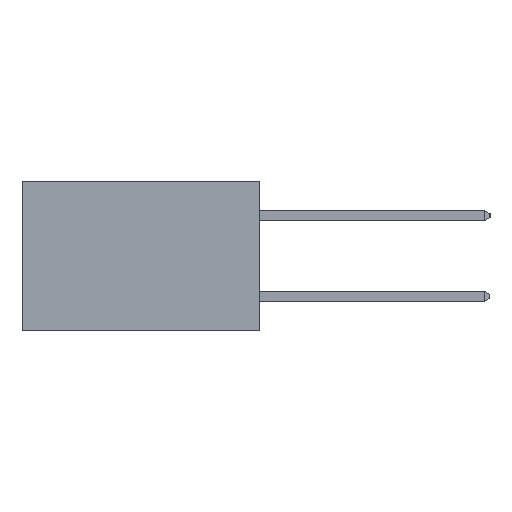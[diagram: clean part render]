
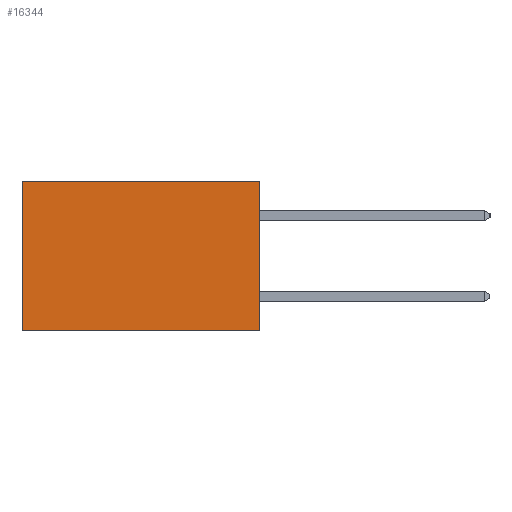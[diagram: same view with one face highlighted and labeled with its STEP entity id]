
A CAD part, left-side view. The second image highlights one B-rep face of the part: STEP entity #16344.
In plain terms, the highlighted planar face has unit normal (-1, 0, 0).
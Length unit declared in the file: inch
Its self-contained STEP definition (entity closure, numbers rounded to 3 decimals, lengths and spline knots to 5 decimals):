
#180 = VECTOR ( 'NONE', #19115, 39.37008 ) ;
#1066 = CARTESIAN_POINT ( 'NONE',  ( 0.277, 0.59, -0.37 ) ) ;
#2022 = VERTEX_POINT ( 'NONE', #5059 ) ;
#2050 = ORIENTED_EDGE ( 'NONE', *, *, #21146, .T. ) ;
#2096 = CARTESIAN_POINT ( 'NONE',  ( 0.277, 0., -0.37 ) ) ;
#2317 = DIRECTION ( 'NONE',  ( 1., 0., 0. ) ) ;
#2644 = ORIENTED_EDGE ( 'NONE', *, *, #7442, .F. ) ;
#2750 = ORIENTED_EDGE ( 'NONE', *, *, #17322, .F. ) ;
#3380 = LINE ( 'NONE', #2096, #12938 ) ;
#3506 = DIRECTION ( 'NONE',  ( 0., 1., 0. ) ) ;
#4027 = ORIENTED_EDGE ( 'NONE', *, *, #23613, .T. ) ;
#5059 = CARTESIAN_POINT ( 'NONE',  ( 0.277, 0.59, 0. ) ) ;
#5318 = LINE ( 'NONE', #1066, #19047 ) ;
#7302 = CARTESIAN_POINT ( 'NONE',  ( 0.277, 0., 0. ) ) ;
#7442 = EDGE_CURVE ( 'NONE', #10250, #15735, #20271, .T. ) ;
#9732 = DIRECTION ( 'NONE',  ( 0., 0., -1. ) ) ;
#9875 = CARTESIAN_POINT ( 'NONE',  ( 0.277, 0., -0.37 ) ) ;
#10025 = VECTOR ( 'NONE', #3506, 39.37008 ) ;
#10250 = VERTEX_POINT ( 'NONE', #10329 ) ;
#10329 = CARTESIAN_POINT ( 'NONE',  ( 0.277, 0., -0.37 ) ) ;
#11353 = AXIS2_PLACEMENT_3D ( 'NONE', #13780, #2317, #15671 ) ;
#12938 = VECTOR ( 'NONE', #9732, 39.37008 ) ;
#13780 = CARTESIAN_POINT ( 'NONE',  ( 0.277, 0., -0.37 ) ) ;
#15092 = LINE ( 'NONE', #7302, #10025 ) ;
#15671 = DIRECTION ( 'NONE',  ( 0., 0., -1. ) ) ;
#15735 = VERTEX_POINT ( 'NONE', #22852 ) ;
#15897 = FACE_OUTER_BOUND ( 'NONE', #21923, .T. ) ;
#16344 = ADVANCED_FACE ( 'NONE', ( #15897 ), #22672, .F. ) ;
#16365 = DIRECTION ( 'NONE',  ( 0., 0., -1. ) ) ;
#17322 = EDGE_CURVE ( 'NONE', #20173, #10250, #3380, .T. ) ;
#17335 = CARTESIAN_POINT ( 'NONE',  ( 0.277, 0., 0. ) ) ;
#19047 = VECTOR ( 'NONE', #16365, 39.37008 ) ;
#19115 = DIRECTION ( 'NONE',  ( 0., 1., 0. ) ) ;
#20173 = VERTEX_POINT ( 'NONE', #17335 ) ;
#20271 = LINE ( 'NONE', #9875, #180 ) ;
#21146 = EDGE_CURVE ( 'NONE', #2022, #15735, #5318, .T. ) ;
#21923 = EDGE_LOOP ( 'NONE', ( #2050, #2644, #2750, #4027 ) ) ;
#22672 = PLANE ( 'NONE',  #11353 ) ;
#22852 = CARTESIAN_POINT ( 'NONE',  ( 0.277, 0.59, -0.37 ) ) ;
#23613 = EDGE_CURVE ( 'NONE', #20173, #2022, #15092, .T. ) ;
